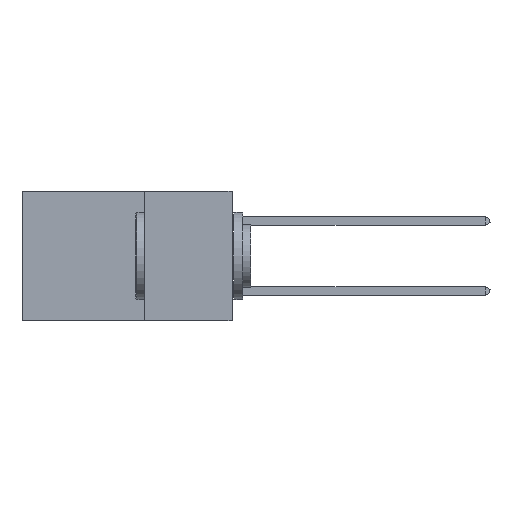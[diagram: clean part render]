
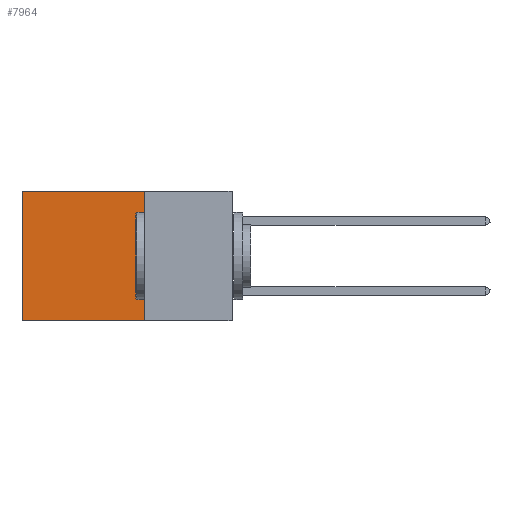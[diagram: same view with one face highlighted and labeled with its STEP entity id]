
A CAD part, left-side view. The second image highlights one B-rep face of the part: STEP entity #7964.
In plain terms, the highlighted planar face has unit normal (-1, 0, 0).
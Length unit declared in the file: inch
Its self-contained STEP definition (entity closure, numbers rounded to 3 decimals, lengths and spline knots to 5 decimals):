
#2535 = LINE ( 'NONE', #4270, #40068 ) ;
#3787 = VERTEX_POINT ( 'NONE', #46216 ) ;
#4270 = CARTESIAN_POINT ( 'NONE',  ( 0.2875, 0.25, 0. ) ) ;
#4457 = VERTEX_POINT ( 'NONE', #27418 ) ;
#5289 = CARTESIAN_POINT ( 'NONE',  ( 0.2875, 0.25, -0.37 ) ) ;
#7826 = EDGE_CURVE ( 'NONE', #3787, #4457, #2535, .T. ) ;
#7964 = ADVANCED_FACE ( 'NONE', ( #36583 ), #34940, .F. ) ;
#11049 = LINE ( 'NONE', #39549, #39680 ) ;
#11257 = VERTEX_POINT ( 'NONE', #17355 ) ;
#11686 = VECTOR ( 'NONE', #17834, 39.37008 ) ;
#11900 = DIRECTION ( 'NONE',  ( 0., 1., 0. ) ) ;
#13076 = EDGE_CURVE ( 'NONE', #11257, #38829, #30369, .T. ) ;
#13458 = DIRECTION ( 'NONE',  ( 0., 0., -1. ) ) ;
#17321 = EDGE_LOOP ( 'NONE', ( #39084, #36779, #24370, #25943 ) ) ;
#17355 = CARTESIAN_POINT ( 'NONE',  ( 0.2875, 0.25, -0.37 ) ) ;
#17834 = DIRECTION ( 'NONE',  ( 0., 0., -1. ) ) ;
#19516 = CARTESIAN_POINT ( 'NONE',  ( 0.2875, 0.6, -0.37 ) ) ;
#21724 = LINE ( 'NONE', #32691, #11686 ) ;
#24370 = ORIENTED_EDGE ( 'NONE', *, *, #25106, .F. ) ;
#25106 = EDGE_CURVE ( 'NONE', #3787, #11257, #21724, .T. ) ;
#25943 = ORIENTED_EDGE ( 'NONE', *, *, #7826, .T. ) ;
#27418 = CARTESIAN_POINT ( 'NONE',  ( 0.2875, 0.6, 0. ) ) ;
#30369 = LINE ( 'NONE', #5289, #37892 ) ;
#31228 = CARTESIAN_POINT ( 'NONE',  ( 0.2875, 0.25, 0. ) ) ;
#32691 = CARTESIAN_POINT ( 'NONE',  ( 0.2875, 0.25, 0. ) ) ;
#34940 = PLANE ( 'NONE',  #41070 ) ;
#36583 = FACE_OUTER_BOUND ( 'NONE', #17321, .T. ) ;
#36779 = ORIENTED_EDGE ( 'NONE', *, *, #13076, .F. ) ;
#37892 = VECTOR ( 'NONE', #39020, 39.37008 ) ;
#38436 = EDGE_CURVE ( 'NONE', #4457, #38829, #11049, .T. ) ;
#38669 = DIRECTION ( 'NONE',  ( 0., 0., -1. ) ) ;
#38829 = VERTEX_POINT ( 'NONE', #19516 ) ;
#39020 = DIRECTION ( 'NONE',  ( 0., 1., 0. ) ) ;
#39084 = ORIENTED_EDGE ( 'NONE', *, *, #38436, .T. ) ;
#39549 = CARTESIAN_POINT ( 'NONE',  ( 0.2875, 0.6, 0. ) ) ;
#39680 = VECTOR ( 'NONE', #13458, 39.37008 ) ;
#40068 = VECTOR ( 'NONE', #11900, 39.37008 ) ;
#41070 = AXIS2_PLACEMENT_3D ( 'NONE', #31228, #42232, #38669 ) ;
#42232 = DIRECTION ( 'NONE',  ( 1., 0., 0. ) ) ;
#46216 = CARTESIAN_POINT ( 'NONE',  ( 0.2875, 0.25, 0. ) ) ;
